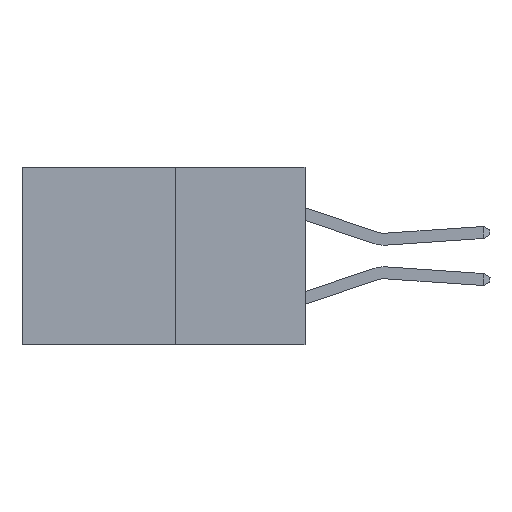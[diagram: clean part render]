
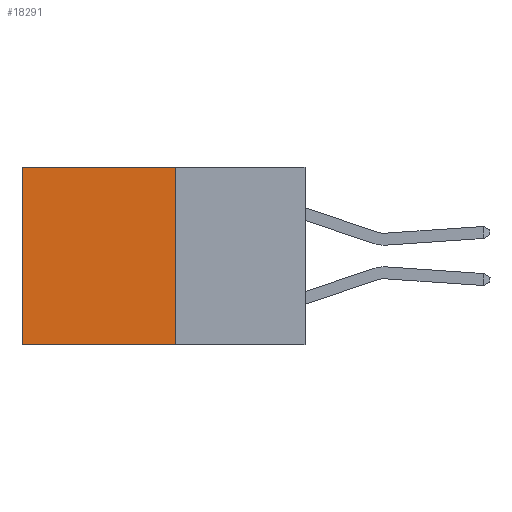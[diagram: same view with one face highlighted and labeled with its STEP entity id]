
A CAD part, left-side view. The second image highlights one B-rep face of the part: STEP entity #18291.
In plain terms, the highlighted planar face has unit normal (-1, 0, 0).
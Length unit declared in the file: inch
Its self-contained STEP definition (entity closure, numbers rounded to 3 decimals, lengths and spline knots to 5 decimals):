
#49 = CARTESIAN_POINT ( 'NONE',  ( 0.277, 0.59, 0. ) ) ;
#226 = AXIS2_PLACEMENT_3D ( 'NONE', #5653, #16019, #7128 ) ;
#884 = VECTOR ( 'NONE', #7446, 39.37008 ) ;
#1432 = VERTEX_POINT ( 'NONE', #49 ) ;
#1640 = VECTOR ( 'NONE', #18251, 39.37008 ) ;
#2654 = VERTEX_POINT ( 'NONE', #18346 ) ;
#2857 = ORIENTED_EDGE ( 'NONE', *, *, #6837, .F. ) ;
#3067 = FACE_OUTER_BOUND ( 'NONE', #8687, .T. ) ;
#3619 = ORIENTED_EDGE ( 'NONE', *, *, #13340, .T. ) ;
#5028 = ORIENTED_EDGE ( 'NONE', *, *, #14095, .F. ) ;
#5653 = CARTESIAN_POINT ( 'NONE',  ( 0.277, 0.27, -0.37 ) ) ;
#5854 = CARTESIAN_POINT ( 'NONE',  ( 0.277, 0.27, -0.37 ) ) ;
#5958 = DIRECTION ( 'NONE',  ( 0., 0., -1. ) ) ;
#6417 = CARTESIAN_POINT ( 'NONE',  ( 0.277, 0.27, -0.37 ) ) ;
#6541 = VERTEX_POINT ( 'NONE', #17681 ) ;
#6837 = EDGE_CURVE ( 'NONE', #2654, #6541, #8048, .T. ) ;
#7128 = DIRECTION ( 'NONE',  ( 0., 0., -1. ) ) ;
#7208 = ORIENTED_EDGE ( 'NONE', *, *, #8749, .T. ) ;
#7446 = DIRECTION ( 'NONE',  ( 0., 0., -1. ) ) ;
#8048 = LINE ( 'NONE', #5854, #11488 ) ;
#8687 = EDGE_LOOP ( 'NONE', ( #3619, #5028, #2857, #7208 ) ) ;
#8749 = EDGE_CURVE ( 'NONE', #2654, #1432, #17031, .T. ) ;
#10304 = CARTESIAN_POINT ( 'NONE',  ( 0.277, 0.59, -0.37 ) ) ;
#10397 = CARTESIAN_POINT ( 'NONE',  ( 0.277, 0.59, -0.37 ) ) ;
#10825 = CARTESIAN_POINT ( 'NONE',  ( 0.277, 0.27, 0. ) ) ;
#11488 = VECTOR ( 'NONE', #5958, 39.37008 ) ;
#12030 = LINE ( 'NONE', #6417, #18996 ) ;
#12732 = VERTEX_POINT ( 'NONE', #10397 ) ;
#12804 = LINE ( 'NONE', #10304, #884 ) ;
#12989 = PLANE ( 'NONE',  #226 ) ;
#13340 = EDGE_CURVE ( 'NONE', #1432, #12732, #12804, .T. ) ;
#14095 = EDGE_CURVE ( 'NONE', #6541, #12732, #12030, .T. ) ;
#16019 = DIRECTION ( 'NONE',  ( 1., 0., 0. ) ) ;
#17031 = LINE ( 'NONE', #10825, #1640 ) ;
#17681 = CARTESIAN_POINT ( 'NONE',  ( 0.277, 0.27, -0.37 ) ) ;
#18220 = DIRECTION ( 'NONE',  ( 0., 1., 0. ) ) ;
#18251 = DIRECTION ( 'NONE',  ( 0., 1., 0. ) ) ;
#18291 = ADVANCED_FACE ( 'NONE', ( #3067 ), #12989, .F. ) ;
#18346 = CARTESIAN_POINT ( 'NONE',  ( 0.277, 0.27, 0. ) ) ;
#18996 = VECTOR ( 'NONE', #18220, 39.37008 ) ;
